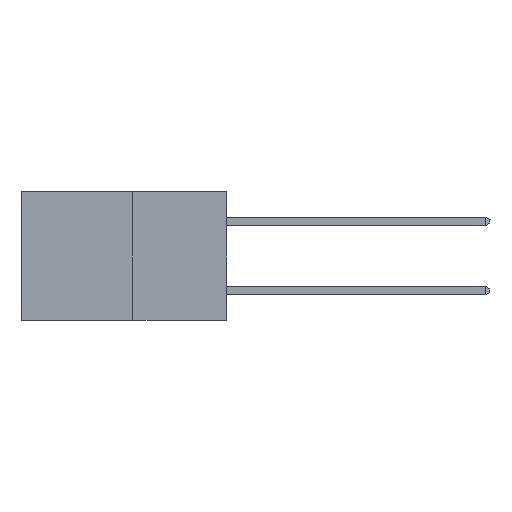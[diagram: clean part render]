
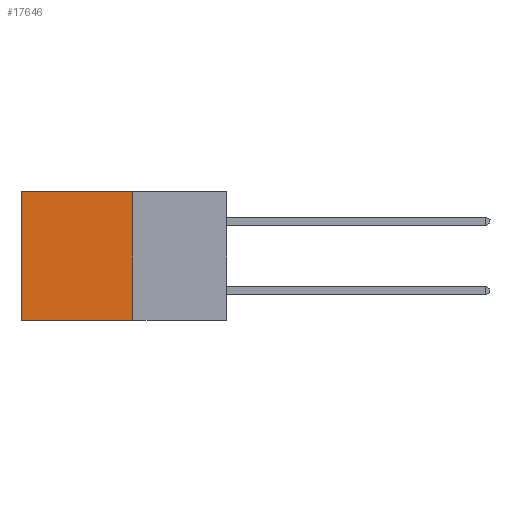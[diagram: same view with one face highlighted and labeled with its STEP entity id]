
A CAD part, left-side view. The second image highlights one B-rep face of the part: STEP entity #17646.
In plain terms, the highlighted planar face has unit normal (-1, 0, 0).
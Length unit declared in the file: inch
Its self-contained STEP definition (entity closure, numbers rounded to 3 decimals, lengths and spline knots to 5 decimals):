
#604 = LINE ( 'NONE', #15000, #16451 ) ;
#821 = CARTESIAN_POINT ( 'NONE',  ( 0.277, 0.59, -0.37 ) ) ;
#1435 = CARTESIAN_POINT ( 'NONE',  ( 0.277, 0.27, 0. ) ) ;
#1880 = DIRECTION ( 'NONE',  ( 1., 0., 0. ) ) ;
#2133 = LINE ( 'NONE', #20029, #24535 ) ;
#2363 = LINE ( 'NONE', #24127, #23486 ) ;
#2758 = VERTEX_POINT ( 'NONE', #1435 ) ;
#4529 = VERTEX_POINT ( 'NONE', #15699 ) ;
#4800 = DIRECTION ( 'NONE',  ( 0., 1., 0. ) ) ;
#8731 = EDGE_CURVE ( 'NONE', #2758, #21680, #604, .T. ) ;
#10421 = ORIENTED_EDGE ( 'NONE', *, *, #18813, .T. ) ;
#10885 = ORIENTED_EDGE ( 'NONE', *, *, #16858, .F. ) ;
#12840 = ORIENTED_EDGE ( 'NONE', *, *, #24904, .F. ) ;
#13632 = EDGE_LOOP ( 'NONE', ( #10421, #12840, #10885, #24564 ) ) ;
#14019 = LINE ( 'NONE', #21663, #24210 ) ;
#14976 = FACE_OUTER_BOUND ( 'NONE', #13632, .T. ) ;
#15000 = CARTESIAN_POINT ( 'NONE',  ( 0.277, 0.27, 0. ) ) ;
#15663 = CARTESIAN_POINT ( 'NONE',  ( 0.277, 0.59, 0. ) ) ;
#15699 = CARTESIAN_POINT ( 'NONE',  ( 0.277, 0.27, -0.37 ) ) ;
#16288 = DIRECTION ( 'NONE',  ( 0., 0., -1. ) ) ;
#16451 = VECTOR ( 'NONE', #4800, 39.37008 ) ;
#16858 = EDGE_CURVE ( 'NONE', #2758, #4529, #2133, .T. ) ;
#17646 = ADVANCED_FACE ( 'NONE', ( #14976 ), #24341, .F. ) ;
#18813 = EDGE_CURVE ( 'NONE', #21680, #26216, #2363, .T. ) ;
#20029 = CARTESIAN_POINT ( 'NONE',  ( 0.277, 0.27, -0.37 ) ) ;
#21663 = CARTESIAN_POINT ( 'NONE',  ( 0.277, 0.27, -0.37 ) ) ;
#21680 = VERTEX_POINT ( 'NONE', #15663 ) ;
#22040 = DIRECTION ( 'NONE',  ( 0., 0., -1. ) ) ;
#22831 = AXIS2_PLACEMENT_3D ( 'NONE', #26369, #1880, #16288 ) ;
#23486 = VECTOR ( 'NONE', #26142, 39.37008 ) ;
#24127 = CARTESIAN_POINT ( 'NONE',  ( 0.277, 0.59, -0.37 ) ) ;
#24210 = VECTOR ( 'NONE', #25704, 39.37008 ) ;
#24341 = PLANE ( 'NONE',  #22831 ) ;
#24535 = VECTOR ( 'NONE', #22040, 39.37008 ) ;
#24564 = ORIENTED_EDGE ( 'NONE', *, *, #8731, .T. ) ;
#24904 = EDGE_CURVE ( 'NONE', #4529, #26216, #14019, .T. ) ;
#25704 = DIRECTION ( 'NONE',  ( 0., 1., 0. ) ) ;
#26142 = DIRECTION ( 'NONE',  ( 0., 0., -1. ) ) ;
#26216 = VERTEX_POINT ( 'NONE', #821 ) ;
#26369 = CARTESIAN_POINT ( 'NONE',  ( 0.277, 0.27, -0.37 ) ) ;
